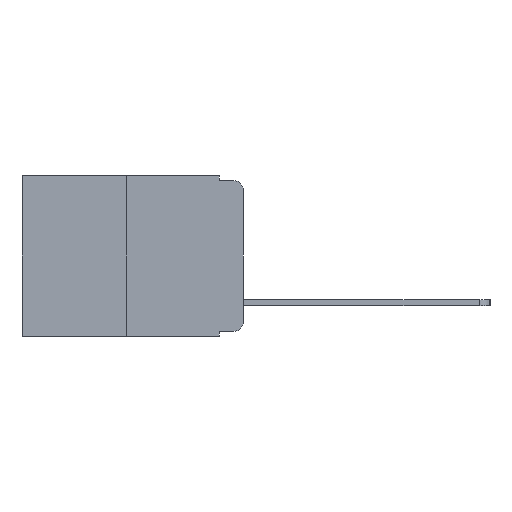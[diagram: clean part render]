
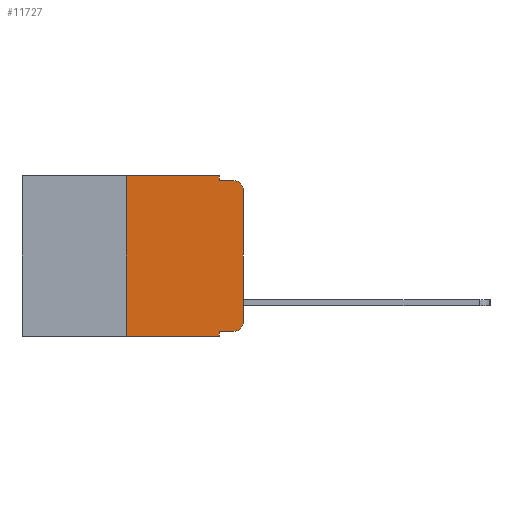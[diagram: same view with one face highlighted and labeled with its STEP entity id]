
A CAD part, left-side view. The second image highlights one B-rep face of the part: STEP entity #11727.
In plain terms, the highlighted planar face has unit normal (-1, 0, 0).
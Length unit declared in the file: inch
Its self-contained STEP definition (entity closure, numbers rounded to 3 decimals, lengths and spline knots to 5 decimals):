
#136 = ORIENTED_EDGE ( 'NONE', *, *, #3594, .T. ) ;
#287 = AXIS2_PLACEMENT_3D ( 'NONE', #2463, #3638, #11508 ) ;
#395 = VERTEX_POINT ( 'NONE', #11513 ) ;
#403 = EDGE_CURVE ( 'NONE', #10388, #6425, #1098, .T. ) ;
#733 = DIRECTION ( 'NONE',  ( 1., 0., 0. ) ) ;
#863 = AXIS2_PLACEMENT_3D ( 'NONE', #5469, #5451, #5423 ) ;
#1098 = LINE ( 'NONE', #1188, #8660 ) ;
#1121 = CARTESIAN_POINT ( 'NONE',  ( 0., 0.25, 0. ) ) ;
#1188 = CARTESIAN_POINT ( 'NONE',  ( 0., 0.473, 0. ) ) ;
#1726 = DIRECTION ( 'NONE',  ( 0., -1., 0. ) ) ;
#2006 = ORIENTED_EDGE ( 'NONE', *, *, #3949, .T. ) ;
#2018 = VERTEX_POINT ( 'NONE', #8451 ) ;
#2230 = LINE ( 'NONE', #8579, #7239 ) ;
#2463 = CARTESIAN_POINT ( 'NONE',  ( 0., 0.02, -0.313 ) ) ;
#2515 = FACE_OUTER_BOUND ( 'NONE', #4549, .T. ) ;
#2573 = VECTOR ( 'NONE', #1726, 39.37008 ) ;
#2883 = VERTEX_POINT ( 'NONE', #5077 ) ;
#2903 = CARTESIAN_POINT ( 'NONE',  ( 0., 0., -0.313 ) ) ;
#3145 = DIRECTION ( 'NONE',  ( 0., -1., 0. ) ) ;
#3154 = VERTEX_POINT ( 'NONE', #4784 ) ;
#3262 = VECTOR ( 'NONE', #7802, 39.37008 ) ;
#3490 = EDGE_CURVE ( 'NONE', #8386, #7689, #5496, .T. ) ;
#3594 = EDGE_CURVE ( 'NONE', #7689, #10360, #8596, .T. ) ;
#3634 = VECTOR ( 'NONE', #12221, 39.37008 ) ;
#3638 = DIRECTION ( 'NONE',  ( -1., 0., 0. ) ) ;
#3723 = ORIENTED_EDGE ( 'NONE', *, *, #3915, .F. ) ;
#3750 = EDGE_CURVE ( 'NONE', #2018, #10360, #11723, .T. ) ;
#3751 = EDGE_CURVE ( 'NONE', #3154, #7211, #2230, .T. ) ;
#3816 = ORIENTED_EDGE ( 'NONE', *, *, #3899, .F. ) ;
#3899 = EDGE_CURVE ( 'NONE', #6425, #2018, #11054, .T. ) ;
#3915 = EDGE_CURVE ( 'NONE', #3154, #10388, #6221, .T. ) ;
#3919 = EDGE_CURVE ( 'NONE', #2883, #7211, #4000, .T. ) ;
#3949 = EDGE_CURVE ( 'NONE', #2883, #395, #10012, .T. ) ;
#3985 = EDGE_CURVE ( 'NONE', #395, #8386, #5350, .T. ) ;
#4000 = LINE ( 'NONE', #4601, #3262 ) ;
#4021 = ORIENTED_EDGE ( 'NONE', *, *, #3751, .T. ) ;
#4402 = DIRECTION ( 'NONE',  ( 0., 0., 1. ) ) ;
#4549 = EDGE_LOOP ( 'NONE', ( #9294, #136, #7898, #3816, #6217, #3723, #4021, #5516, #2006, #6834 ) ) ;
#4601 = CARTESIAN_POINT ( 'NONE',  ( 0., 0.051, 0. ) ) ;
#4704 = CARTESIAN_POINT ( 'NONE',  ( 0., 0.051, -0.343 ) ) ;
#4784 = CARTESIAN_POINT ( 'NONE',  ( 0., 0.25, -0.343 ) ) ;
#5049 = PLANE ( 'NONE',  #8592 ) ;
#5077 = CARTESIAN_POINT ( 'NONE',  ( 0., 0.051, -0.333 ) ) ;
#5209 = VECTOR ( 'NONE', #8096, 39.37008 ) ;
#5320 = CARTESIAN_POINT ( 'NONE',  ( 0., 0.25, 0. ) ) ;
#5350 = CIRCLE ( 'NONE', #287, 0.02 ) ;
#5423 = DIRECTION ( 'NONE',  ( 0., 0., -1. ) ) ;
#5451 = DIRECTION ( 'NONE',  ( -1., 0., 0. ) ) ;
#5469 = CARTESIAN_POINT ( 'NONE',  ( 0., 0.02, -0.03 ) ) ;
#5496 = LINE ( 'NONE', #8044, #5209 ) ;
#5516 = ORIENTED_EDGE ( 'NONE', *, *, #3919, .F. ) ;
#6217 = ORIENTED_EDGE ( 'NONE', *, *, #403, .F. ) ;
#6221 = LINE ( 'NONE', #5320, #8332 ) ;
#6425 = VERTEX_POINT ( 'NONE', #11828 ) ;
#6834 = ORIENTED_EDGE ( 'NONE', *, *, #3985, .T. ) ;
#6914 = CARTESIAN_POINT ( 'NONE',  ( 0., 0.473, 0. ) ) ;
#7029 = DIRECTION ( 'NONE',  ( 0., -1., 0. ) ) ;
#7211 = VERTEX_POINT ( 'NONE', #4704 ) ;
#7239 = VECTOR ( 'NONE', #7029, 39.37008 ) ;
#7522 = VECTOR ( 'NONE', #8608, 39.37008 ) ;
#7689 = VERTEX_POINT ( 'NONE', #11761 ) ;
#7802 = DIRECTION ( 'NONE',  ( 0., 0., -1. ) ) ;
#7821 = DIRECTION ( 'NONE',  ( 0., 0., -1. ) ) ;
#7898 = ORIENTED_EDGE ( 'NONE', *, *, #3750, .F. ) ;
#8044 = CARTESIAN_POINT ( 'NONE',  ( 0., 0., 0. ) ) ;
#8096 = DIRECTION ( 'NONE',  ( 0., 0., 1. ) ) ;
#8332 = VECTOR ( 'NONE', #4402, 39.37008 ) ;
#8386 = VERTEX_POINT ( 'NONE', #2903 ) ;
#8451 = CARTESIAN_POINT ( 'NONE',  ( 0., 0.051, -0.01 ) ) ;
#8579 = CARTESIAN_POINT ( 'NONE',  ( 0., 0.473, -0.343 ) ) ;
#8592 = AXIS2_PLACEMENT_3D ( 'NONE', #6914, #733, #7821 ) ;
#8596 = CIRCLE ( 'NONE', #863, 0.02 ) ;
#8608 = DIRECTION ( 'NONE',  ( 0., -1., 0. ) ) ;
#8624 = CARTESIAN_POINT ( 'NONE',  ( 0., 0.051, -0.01 ) ) ;
#8660 = VECTOR ( 'NONE', #3145, 39.37008 ) ;
#9294 = ORIENTED_EDGE ( 'NONE', *, *, #3490, .T. ) ;
#10012 = LINE ( 'NONE', #12028, #2573 ) ;
#10296 = CARTESIAN_POINT ( 'NONE',  ( 0., 0.02, -0.01 ) ) ;
#10360 = VERTEX_POINT ( 'NONE', #10296 ) ;
#10388 = VERTEX_POINT ( 'NONE', #1121 ) ;
#11054 = LINE ( 'NONE', #12256, #3634 ) ;
#11508 = DIRECTION ( 'NONE',  ( 0., 0., -1. ) ) ;
#11513 = CARTESIAN_POINT ( 'NONE',  ( 0., 0.02, -0.333 ) ) ;
#11723 = LINE ( 'NONE', #8624, #7522 ) ;
#11727 = ADVANCED_FACE ( 'NONE', ( #2515 ), #5049, .F. ) ;
#11761 = CARTESIAN_POINT ( 'NONE',  ( 0., 0., -0.03 ) ) ;
#11828 = CARTESIAN_POINT ( 'NONE',  ( 0., 0.051, 0. ) ) ;
#12028 = CARTESIAN_POINT ( 'NONE',  ( 0., 0.051, -0.333 ) ) ;
#12221 = DIRECTION ( 'NONE',  ( 0., 0., -1. ) ) ;
#12256 = CARTESIAN_POINT ( 'NONE',  ( 0., 0.051, 0. ) ) ;
